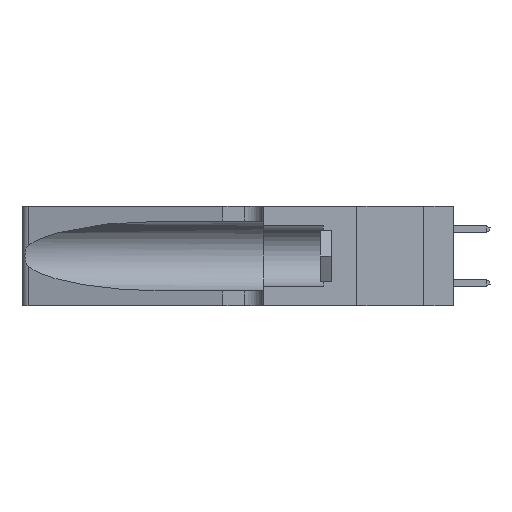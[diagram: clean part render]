
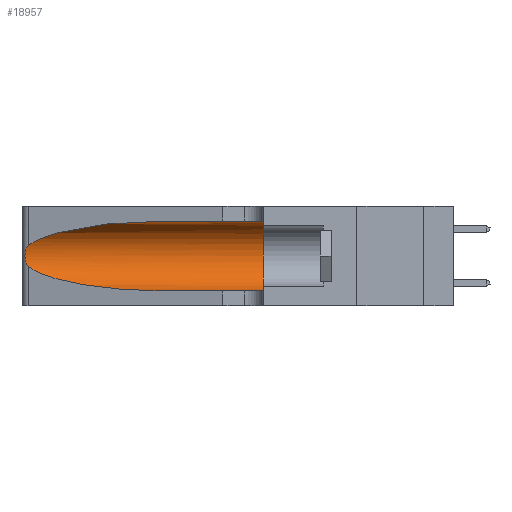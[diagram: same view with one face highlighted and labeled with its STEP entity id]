
A CAD part, left-side view. The second image highlights one B-rep face of the part: STEP entity #18957.
In plain terms, the highlighted cylindrical face has radius 3.308 mm (diameter 6.617 mm), a partial arc.
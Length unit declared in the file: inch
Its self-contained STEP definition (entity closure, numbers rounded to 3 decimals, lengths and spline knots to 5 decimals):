
#114 = CARTESIAN_POINT ( 'NONE',  ( 0.25487, 1.22718, 0.22369 ) ) ;
#238 = CARTESIAN_POINT ( 'NONE',  ( 0.25487, 1.22718, 0.14631 ) ) ;
#412 = ORIENTED_EDGE ( 'NONE', *, *, #35226, .F. ) ;
#893 = CARTESIAN_POINT ( 'NONE',  ( 0.25487, 1.22718, 0.14631 ) ) ;
#937 = CARTESIAN_POINT ( 'NONE',  ( 0.1305, 1.61858, 0.05475 ) ) ;
#1012 = EDGE_CURVE ( 'NONE', #28561, #10916, #31529, .T. ) ;
#3117 = CARTESIAN_POINT ( 'NONE',  ( 0.25639, 1.23184, 0.21858 ) ) ;
#4012 = CARTESIAN_POINT ( 'NONE',  ( 0.1305, 0.72297, 0.05475 ) ) ;
#4165 = LINE ( 'NONE', #22566, #34389 ) ;
#4178 = DIRECTION ( 'NONE',  ( 0., 1., 0. ) ) ;
#4831 = VECTOR ( 'NONE', #6829, 39.37008 ) ;
#5101 = FACE_OUTER_BOUND ( 'NONE', #18148, .T. ) ;
#5120 = ORIENTED_EDGE ( 'NONE', *, *, #37409, .T. ) ;
#6096 = CARTESIAN_POINT ( 'NONE',  ( 0.25854, 1.2359, 0.20912 ) ) ;
#6143 = CARTESIAN_POINT ( 'NONE',  ( 0.1305, 1.61858, 0.185 ) ) ;
#6355 = EDGE_CURVE ( 'NONE', #9922, #21425, #20106, .T. ) ;
#6829 = DIRECTION ( 'NONE',  ( 0., -1., 0. ) ) ;
#7387 = CARTESIAN_POINT ( 'NONE',  ( 0.1305, 0.35, 0.31525 ) ) ;
#7698 = ORIENTED_EDGE ( 'NONE', *, *, #29162, .T. ) ;
#8352 =( BOUNDED_CURVE ( )  B_SPLINE_CURVE ( 3, ( #893, #33228, #21755, #4012 ),
 .UNSPECIFIED., .F., .T. ) 
 B_SPLINE_CURVE_WITH_KNOTS ( ( 4, 4 ),
 ( 3.44316, 4.71239 ),
 .UNSPECIFIED. ) 
 CURVE ( )  GEOMETRIC_REPRESENTATION_ITEM ( )  RATIONAL_B_SPLINE_CURVE ( ( 1., 0.87, 0.87, 1. ) ) 
 REPRESENTATION_ITEM ( '' )  );
#8479 = CARTESIAN_POINT ( 'NONE',  ( 0.1305, 0.72297, 0.05475 ) ) ;
#9115 = CARTESIAN_POINT ( 'NONE',  ( 0.26075, 1.23896, 0.19203 ) ) ;
#9922 = VERTEX_POINT ( 'NONE', #7387 ) ;
#10916 = VERTEX_POINT ( 'NONE', #26974 ) ;
#12108 = CARTESIAN_POINT ( 'NONE',  ( 0.26017, 1.23833, 0.17102 ) ) ;
#15078 = CARTESIAN_POINT ( 'NONE',  ( 0.25789, 1.23486, 0.15765 ) ) ;
#16309 = ORIENTED_EDGE ( 'NONE', *, *, #1012, .T. ) ;
#18024 = CARTESIAN_POINT ( 'NONE',  ( 0.25555, 1.22993, 0.14849 ) ) ;
#18072 = DIRECTION ( 'NONE',  ( 0., 0., -1. ) ) ;
#18148 = EDGE_LOOP ( 'NONE', ( #16309, #5120, #7698, #35526, #23347, #412 ) ) ;
#18957 = ADVANCED_FACE ( 'NONE', ( #5101 ), #34390, .F. ) ;
#19245 = CARTESIAN_POINT ( 'NONE',  ( 0.1305, 0.72297, 0.31525 ) ) ;
#19768 = DIRECTION ( 'NONE',  ( 0., -1., 0. ) ) ;
#20106 = CIRCLE ( 'NONE', #37657, 0.13025 ) ;
#20612 = LINE ( 'NONE', #937, #4831 ) ;
#21425 = VERTEX_POINT ( 'NONE', #33699 ) ;
#21755 = CARTESIAN_POINT ( 'NONE',  ( 0.18966, 0.96281, 0.05475 ) ) ;
#21915 = CARTESIAN_POINT ( 'NONE',  ( 0.1305, 0.35, 0.185 ) ) ;
#22566 = CARTESIAN_POINT ( 'NONE',  ( 0.1305, 1.61858, 0.31525 ) ) ;
#23347 = ORIENTED_EDGE ( 'NONE', *, *, #6355, .F. ) ;
#23798 = CARTESIAN_POINT ( 'NONE',  ( 0.25787, 1.23484, 0.2124 ) ) ;
#24835 = DIRECTION ( 'NONE',  ( 0., 0., 1. ) ) ;
#26031 = B_SPLINE_CURVE_WITH_KNOTS ( 'NONE', 3,
 ( #114, #35238, #3117, #23798, #6096, #26697, #9115, #29552, #12108, #32445, #15078, #35357, #18024, #238 ),
 .UNSPECIFIED., .F., .F.,
 ( 4, 2, 2, 2, 2, 2, 4 ),
 ( 0., 0.00027, 0.00053, 0.00107, 0.0016, 0.00187, 0.00214 ),
 .UNSPECIFIED. ) ;
#26306 = VERTEX_POINT ( 'NONE', #8479 ) ;
#26697 = CARTESIAN_POINT ( 'NONE',  ( 0.26018, 1.23835, 0.19895 ) ) ;
#26974 = CARTESIAN_POINT ( 'NONE',  ( 0.25487, 1.22718, 0.22369 ) ) ;
#28561 = VERTEX_POINT ( 'NONE', #19245 ) ;
#29162 = EDGE_CURVE ( 'NONE', #33842, #26306, #8352, .T. ) ;
#29552 = CARTESIAN_POINT ( 'NONE',  ( 0.26075, 1.23896, 0.178 ) ) ;
#29941 = CARTESIAN_POINT ( 'NONE',  ( 0.1305, 0.72297, 0.31525 ) ) ;
#30013 = CARTESIAN_POINT ( 'NONE',  ( 0.18966, 0.96281, 0.31525 ) ) ;
#30605 = CARTESIAN_POINT ( 'NONE',  ( 0.25487, 1.22718, 0.22369 ) ) ;
#30675 = CARTESIAN_POINT ( 'NONE',  ( 0.25487, 1.22718, 0.14631 ) ) ;
#31529 =( BOUNDED_CURVE ( )  B_SPLINE_CURVE ( 3, ( #29941, #30013, #36762, #30605 ),
 .UNSPECIFIED., .F., .F. ) 
 B_SPLINE_CURVE_WITH_KNOTS ( ( 4, 4 ),
 ( 1.5708, 2.84003 ),
 .UNSPECIFIED. ) 
 CURVE ( )  GEOMETRIC_REPRESENTATION_ITEM ( )  RATIONAL_B_SPLINE_CURVE ( ( 1., 0.87, 0.87, 1. ) ) 
 REPRESENTATION_ITEM ( '' )  );
#32445 = CARTESIAN_POINT ( 'NONE',  ( 0.25856, 1.23593, 0.16098 ) ) ;
#32497 = DIRECTION ( 'NONE',  ( 0., -1., 0. ) ) ;
#33074 = EDGE_CURVE ( 'NONE', #26306, #21425, #20612, .T. ) ;
#33228 = CARTESIAN_POINT ( 'NONE',  ( 0.2373, 1.15595, 0.08982 ) ) ;
#33699 = CARTESIAN_POINT ( 'NONE',  ( 0.1305, 0.35, 0.05475 ) ) ;
#33842 = VERTEX_POINT ( 'NONE', #30675 ) ;
#34389 = VECTOR ( 'NONE', #19768, 39.37008 ) ;
#34390 = CYLINDRICAL_SURFACE ( 'NONE', #35454, 0.13025 ) ;
#35226 = EDGE_CURVE ( 'NONE', #28561, #9922, #4165, .T. ) ;
#35238 = CARTESIAN_POINT ( 'NONE',  ( 0.25555, 1.22994, 0.2215 ) ) ;
#35357 = CARTESIAN_POINT ( 'NONE',  ( 0.25639, 1.23186, 0.15144 ) ) ;
#35454 = AXIS2_PLACEMENT_3D ( 'NONE', #6143, #32497, #18072 ) ;
#35526 = ORIENTED_EDGE ( 'NONE', *, *, #33074, .T. ) ;
#36762 = CARTESIAN_POINT ( 'NONE',  ( 0.2373, 1.15595, 0.28018 ) ) ;
#37409 = EDGE_CURVE ( 'NONE', #10916, #33842, #26031, .T. ) ;
#37657 = AXIS2_PLACEMENT_3D ( 'NONE', #21915, #4178, #24835 ) ;
